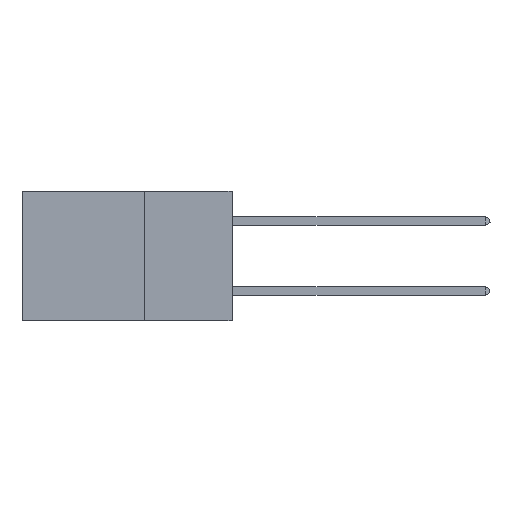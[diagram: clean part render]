
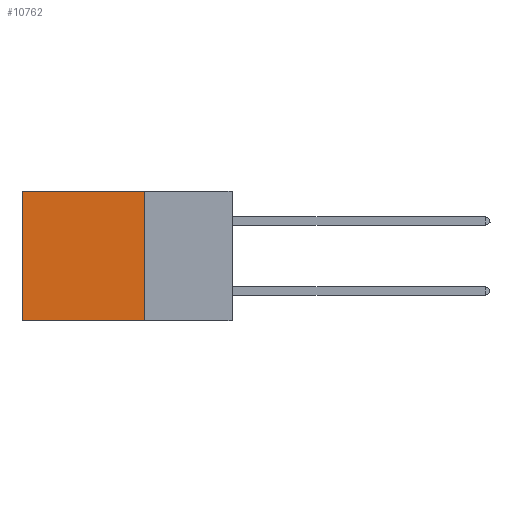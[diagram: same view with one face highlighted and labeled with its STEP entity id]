
A CAD part, left-side view. The second image highlights one B-rep face of the part: STEP entity #10762.
In plain terms, the highlighted planar face has unit normal (-1, 0, 0).
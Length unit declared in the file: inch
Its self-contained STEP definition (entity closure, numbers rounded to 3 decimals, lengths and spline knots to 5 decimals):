
#4532 = EDGE_CURVE ( 'NONE', #33862, #24318, #8095, .T. ) ;
#4668 = DIRECTION ( 'NONE',  ( 0., 0., -1. ) ) ;
#4685 = DIRECTION ( 'NONE',  ( 0., 0., -1. ) ) ;
#6247 = AXIS2_PLACEMENT_3D ( 'NONE', #21660, #32185, #8553 ) ;
#8095 = LINE ( 'NONE', #28315, #16736 ) ;
#8553 = DIRECTION ( 'NONE',  ( 0., 0., -1. ) ) ;
#8724 = VECTOR ( 'NONE', #26474, 39.37008 ) ;
#9468 = VECTOR ( 'NONE', #21927, 39.37008 ) ;
#10762 = ADVANCED_FACE ( 'NONE', ( #26863 ), #29599, .F. ) ;
#10816 = VERTEX_POINT ( 'NONE', #33212 ) ;
#14245 = ORIENTED_EDGE ( 'NONE', *, *, #4532, .F. ) ;
#15520 = CARTESIAN_POINT ( 'NONE',  ( 0.2875, 0.6, -0.37 ) ) ;
#15764 = ORIENTED_EDGE ( 'NONE', *, *, #23214, .F. ) ;
#15786 = CARTESIAN_POINT ( 'NONE',  ( 0.2875, 0.25, 0. ) ) ;
#16323 = EDGE_CURVE ( 'NONE', #10816, #17684, #28295, .T. ) ;
#16736 = VECTOR ( 'NONE', #4685, 39.37008 ) ;
#16935 = LINE ( 'NONE', #21754, #9468 ) ;
#17684 = VERTEX_POINT ( 'NONE', #15520 ) ;
#18658 = EDGE_CURVE ( 'NONE', #33862, #10816, #21293, .T. ) ;
#19691 = EDGE_LOOP ( 'NONE', ( #21126, #15764, #14245, #31672 ) ) ;
#21126 = ORIENTED_EDGE ( 'NONE', *, *, #16323, .T. ) ;
#21293 = LINE ( 'NONE', #15786, #8724 ) ;
#21660 = CARTESIAN_POINT ( 'NONE',  ( 0.2875, 0.25, 0. ) ) ;
#21754 = CARTESIAN_POINT ( 'NONE',  ( 0.2875, 0.25, -0.37 ) ) ;
#21927 = DIRECTION ( 'NONE',  ( 0., 1., 0. ) ) ;
#23214 = EDGE_CURVE ( 'NONE', #24318, #17684, #16935, .T. ) ;
#24318 = VERTEX_POINT ( 'NONE', #26798 ) ;
#24656 = CARTESIAN_POINT ( 'NONE',  ( 0.2875, 0.25, 0. ) ) ;
#24697 = VECTOR ( 'NONE', #4668, 39.37008 ) ;
#26474 = DIRECTION ( 'NONE',  ( 0., 1., 0. ) ) ;
#26798 = CARTESIAN_POINT ( 'NONE',  ( 0.2875, 0.25, -0.37 ) ) ;
#26863 = FACE_OUTER_BOUND ( 'NONE', #19691, .T. ) ;
#28295 = LINE ( 'NONE', #28461, #24697 ) ;
#28315 = CARTESIAN_POINT ( 'NONE',  ( 0.2875, 0.25, 0. ) ) ;
#28461 = CARTESIAN_POINT ( 'NONE',  ( 0.2875, 0.6, 0. ) ) ;
#29599 = PLANE ( 'NONE',  #6247 ) ;
#31672 = ORIENTED_EDGE ( 'NONE', *, *, #18658, .T. ) ;
#32185 = DIRECTION ( 'NONE',  ( 1., 0., 0. ) ) ;
#33212 = CARTESIAN_POINT ( 'NONE',  ( 0.2875, 0.6, 0. ) ) ;
#33862 = VERTEX_POINT ( 'NONE', #24656 ) ;
